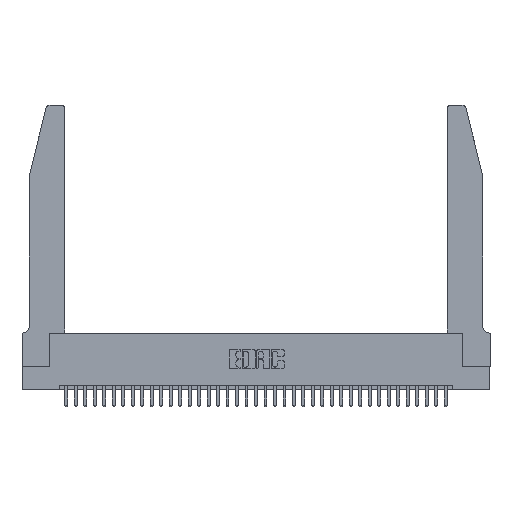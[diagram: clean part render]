
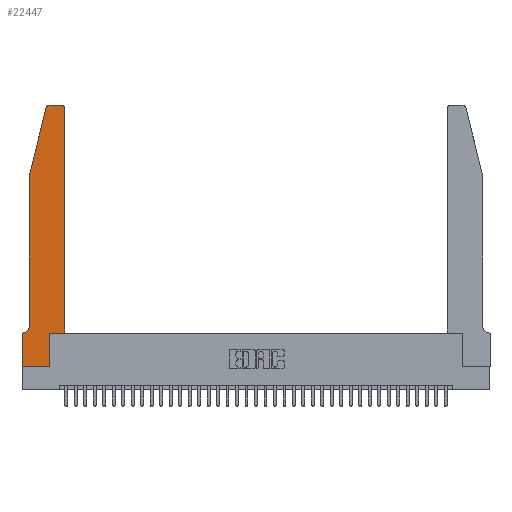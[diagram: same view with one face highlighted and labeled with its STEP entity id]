
A CAD part, top view. The second image highlights one B-rep face of the part: STEP entity #22447.
In plain terms, the highlighted planar face has unit normal (0, 0, 1).
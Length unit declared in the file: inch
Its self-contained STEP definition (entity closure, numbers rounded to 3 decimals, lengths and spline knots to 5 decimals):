
#371 = LINE ( 'NONE', #36433, #30095 ) ;
#1035 = EDGE_CURVE ( 'NONE', #10570, #31646, #371, .T. ) ;
#1414 = EDGE_CURVE ( 'NONE', #5180, #4727, #8933, .T. ) ;
#1667 = VERTEX_POINT ( 'NONE', #25056 ) ;
#2563 = LINE ( 'NONE', #7408, #29919 ) ;
#3110 = ORIENTED_EDGE ( 'NONE', *, *, #17154, .T. ) ;
#3243 = DIRECTION ( 'NONE',  ( 1., 0., 0. ) ) ;
#3477 = VECTOR ( 'NONE', #37164, 39.37008 ) ;
#3577 = AXIS2_PLACEMENT_3D ( 'NONE', #29630, #9501, #18262 ) ;
#4004 = CARTESIAN_POINT ( 'NONE',  ( 0.284, 2.72, 0.37 ) ) ;
#4601 = LINE ( 'NONE', #13516, #32407 ) ;
#4694 = ORIENTED_EDGE ( 'NONE', *, *, #1414, .T. ) ;
#4727 = VERTEX_POINT ( 'NONE', #27847 ) ;
#5180 = VERTEX_POINT ( 'NONE', #31032 ) ;
#5478 = VECTOR ( 'NONE', #36709, 39.37008 ) ;
#5623 = CARTESIAN_POINT ( 'NONE',  ( 0.0755, 0.35, 0.37 ) ) ;
#6329 = VECTOR ( 'NONE', #3243, 39.37008 ) ;
#6497 = EDGE_CURVE ( 'NONE', #13461, #23160, #33572, .T. ) ;
#6843 = CARTESIAN_POINT ( 'NONE',  ( 0.2865, 0.35, 0.37 ) ) ;
#7032 = DIRECTION ( 'NONE',  ( 0., 0., 1. ) ) ;
#7142 = DIRECTION ( 'NONE',  ( 0., -1., 0. ) ) ;
#7408 = CARTESIAN_POINT ( 'NONE',  ( 0.0755, 2., 0.37 ) ) ;
#7813 = EDGE_CURVE ( 'NONE', #26704, #21091, #34777, .T. ) ;
#8434 = ORIENTED_EDGE ( 'NONE', *, *, #9346, .T. ) ;
#8480 = VERTEX_POINT ( 'NONE', #21071 ) ;
#8933 = LINE ( 'NONE', #24190, #11187 ) ;
#9346 = EDGE_CURVE ( 'NONE', #1667, #30345, #10825, .T. ) ;
#9350 = CARTESIAN_POINT ( 'NONE',  ( 0.4505, 0.35, 0.37 ) ) ;
#9501 = DIRECTION ( 'NONE',  ( 0., 0., 1. ) ) ;
#9871 = VECTOR ( 'NONE', #36162, 39.37008 ) ;
#10010 = CARTESIAN_POINT ( 'NONE',  ( 0.2605, 2.75, 0.37 ) ) ;
#10187 = ORIENTED_EDGE ( 'NONE', *, *, #6497, .T. ) ;
#10352 = LINE ( 'NONE', #9350, #9871 ) ;
#10570 = VERTEX_POINT ( 'NONE', #22105 ) ;
#10825 = LINE ( 'NONE', #10010, #5478 ) ;
#11051 = FACE_OUTER_BOUND ( 'NONE', #25100, .T. ) ;
#11187 = VECTOR ( 'NONE', #24315, 39.37008 ) ;
#11363 = AXIS2_PLACEMENT_3D ( 'NONE', #33154, #24876, #27760 ) ;
#11575 = DIRECTION ( 'NONE',  ( 0., 1., 0. ) ) ;
#13461 = VERTEX_POINT ( 'NONE', #16698 ) ;
#13516 = CARTESIAN_POINT ( 'NONE',  ( 0., 0., 0.37 ) ) ;
#14006 = CARTESIAN_POINT ( 'NONE',  ( 0.2865, 0.35, 0.37 ) ) ;
#14338 = EDGE_CURVE ( 'NONE', #21091, #10570, #10352, .T. ) ;
#15166 = DIRECTION ( 'NONE',  ( 0., 1., 0. ) ) ;
#15357 = ORIENTED_EDGE ( 'NONE', *, *, #7813, .T. ) ;
#15449 = CIRCLE ( 'NONE', #3577, 0.03 ) ;
#15820 = CARTESIAN_POINT ( 'NONE',  ( 0.0055, 0.42, 0.37 ) ) ;
#16698 = CARTESIAN_POINT ( 'NONE',  ( 0.0755, 0.42, 0.37 ) ) ;
#17154 = EDGE_CURVE ( 'NONE', #30345, #5180, #37199, .T. ) ;
#17714 = EDGE_CURVE ( 'NONE', #4727, #13461, #2563, .T. ) ;
#17950 = ORIENTED_EDGE ( 'NONE', *, *, #33169, .T. ) ;
#18076 = VECTOR ( 'NONE', #11575, 39.37008 ) ;
#18262 = DIRECTION ( 'NONE',  ( 1., 0., 0. ) ) ;
#18673 = DIRECTION ( 'NONE',  ( -1., 0., 0. ) ) ;
#19024 = PLANE ( 'NONE',  #11363 ) ;
#20763 = VERTEX_POINT ( 'NONE', #34037 ) ;
#21071 = CARTESIAN_POINT ( 'NONE',  ( 0., 0., 0.37 ) ) ;
#21091 = VERTEX_POINT ( 'NONE', #6843 ) ;
#21826 = CARTESIAN_POINT ( 'NONE',  ( 0.0055, 0.35, 0.37 ) ) ;
#22105 = CARTESIAN_POINT ( 'NONE',  ( 0.4505, 0.35, 0.37 ) ) ;
#22447 = ADVANCED_FACE ( 'NONE', ( #11051 ), #19024, .T. ) ;
#23160 = VERTEX_POINT ( 'NONE', #21826 ) ;
#23255 = LINE ( 'NONE', #5623, #3477 ) ;
#23971 = CARTESIAN_POINT ( 'NONE',  ( 0.4505, 2.72, 0.37 ) ) ;
#24092 = DIRECTION ( 'NONE',  ( 1., 0., 0. ) ) ;
#24106 = EDGE_CURVE ( 'NONE', #8480, #26704, #31169, .T. ) ;
#24190 = CARTESIAN_POINT ( 'NONE',  ( 0.0755, 2., 0.37 ) ) ;
#24315 = DIRECTION ( 'NONE',  ( -0.239, -0.971, 0. ) ) ;
#24522 = EDGE_CURVE ( 'NONE', #20763, #8480, #4601, .T. ) ;
#24876 = DIRECTION ( 'NONE',  ( 0., 0., 1. ) ) ;
#25056 = CARTESIAN_POINT ( 'NONE',  ( 0.4205, 2.75, 0.37 ) ) ;
#25100 = EDGE_LOOP ( 'NONE', ( #8434, #3110, #4694, #37008, #10187, #17950, #35908, #30736, #15357, #28204, #34597, #26927 ) ) ;
#26704 = VERTEX_POINT ( 'NONE', #28094 ) ;
#26927 = ORIENTED_EDGE ( 'NONE', *, *, #32054, .T. ) ;
#27532 = AXIS2_PLACEMENT_3D ( 'NONE', #15820, #35958, #18673 ) ;
#27760 = DIRECTION ( 'NONE',  ( 1., 0., 0. ) ) ;
#27847 = CARTESIAN_POINT ( 'NONE',  ( 0.0755, 2., 0.37 ) ) ;
#28094 = CARTESIAN_POINT ( 'NONE',  ( 0.2865, 0., 0.37 ) ) ;
#28204 = ORIENTED_EDGE ( 'NONE', *, *, #14338, .T. ) ;
#29630 = CARTESIAN_POINT ( 'NONE',  ( 0.4205, 2.72, 0.37 ) ) ;
#29891 = CARTESIAN_POINT ( 'NONE',  ( 0.284, 2.75, 0.37 ) ) ;
#29919 = VECTOR ( 'NONE', #7142, 39.37008 ) ;
#30095 = VECTOR ( 'NONE', #15166, 39.37008 ) ;
#30345 = VERTEX_POINT ( 'NONE', #29891 ) ;
#30736 = ORIENTED_EDGE ( 'NONE', *, *, #24106, .T. ) ;
#31032 = CARTESIAN_POINT ( 'NONE',  ( 0.25487, 2.72718, 0.37 ) ) ;
#31169 = LINE ( 'NONE', #37187, #6329 ) ;
#31646 = VERTEX_POINT ( 'NONE', #23971 ) ;
#32054 = EDGE_CURVE ( 'NONE', #31646, #1667, #15449, .T. ) ;
#32083 = AXIS2_PLACEMENT_3D ( 'NONE', #4004, #7032, #24092 ) ;
#32407 = VECTOR ( 'NONE', #36665, 39.37008 ) ;
#33154 = CARTESIAN_POINT ( 'NONE',  ( 0., 0.35, 0.37 ) ) ;
#33169 = EDGE_CURVE ( 'NONE', #23160, #20763, #23255, .T. ) ;
#33572 = CIRCLE ( 'NONE', #27532, 0.07 ) ;
#34037 = CARTESIAN_POINT ( 'NONE',  ( 0., 0.35, 0.37 ) ) ;
#34597 = ORIENTED_EDGE ( 'NONE', *, *, #1035, .T. ) ;
#34777 = LINE ( 'NONE', #14006, #18076 ) ;
#35908 = ORIENTED_EDGE ( 'NONE', *, *, #24522, .T. ) ;
#35958 = DIRECTION ( 'NONE',  ( 0., 0., -1. ) ) ;
#36162 = DIRECTION ( 'NONE',  ( 1., 0., 0. ) ) ;
#36433 = CARTESIAN_POINT ( 'NONE',  ( 0.4505, 0.35, 0.37 ) ) ;
#36665 = DIRECTION ( 'NONE',  ( 0., -1., 0. ) ) ;
#36709 = DIRECTION ( 'NONE',  ( -1., 0., 0. ) ) ;
#37008 = ORIENTED_EDGE ( 'NONE', *, *, #17714, .T. ) ;
#37164 = DIRECTION ( 'NONE',  ( -1., 0., 0. ) ) ;
#37187 = CARTESIAN_POINT ( 'NONE',  ( 0., 0., 0.37 ) ) ;
#37199 = CIRCLE ( 'NONE', #32083, 0.03 ) ;
